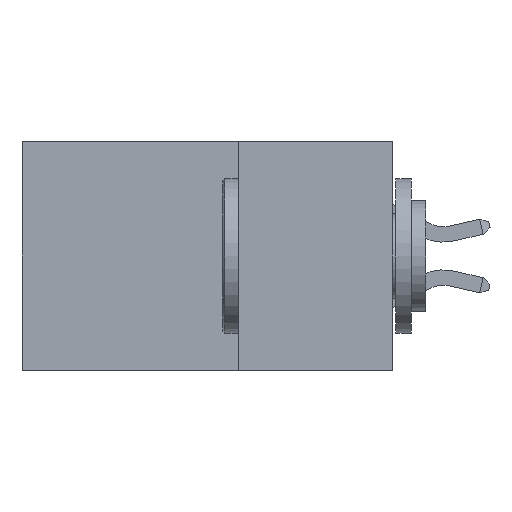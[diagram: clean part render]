
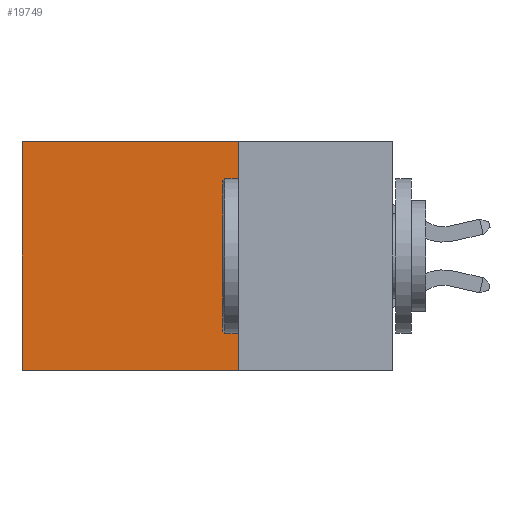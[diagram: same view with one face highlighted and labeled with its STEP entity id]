
A CAD part, left-side view. The second image highlights one B-rep face of the part: STEP entity #19749.
In plain terms, the highlighted planar face has unit normal (-1, 0, 0).
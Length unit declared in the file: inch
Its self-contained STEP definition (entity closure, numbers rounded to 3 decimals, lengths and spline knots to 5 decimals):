
#245 = LINE ( 'NONE', #20423, #14834 ) ;
#552 = CARTESIAN_POINT ( 'NONE',  ( 0.2875, 0.25, 0. ) ) ;
#1930 = DIRECTION ( 'NONE',  ( 0., 0., -1. ) ) ;
#2549 = CARTESIAN_POINT ( 'NONE',  ( 0.2875, 0.6, -0.37 ) ) ;
#3385 = EDGE_CURVE ( 'NONE', #13468, #19753, #19648, .T. ) ;
#4833 = EDGE_CURVE ( 'NONE', #16592, #5037, #22550, .T. ) ;
#4942 = DIRECTION ( 'NONE',  ( 0., 1., 0. ) ) ;
#5016 = EDGE_CURVE ( 'NONE', #13468, #16592, #245, .T. ) ;
#5037 = VERTEX_POINT ( 'NONE', #2549 ) ;
#5762 = DIRECTION ( 'NONE',  ( 1., 0., 0. ) ) ;
#8486 = DIRECTION ( 'NONE',  ( 0., 0., -1. ) ) ;
#8752 = CARTESIAN_POINT ( 'NONE',  ( 0.2875, 0.6, 0. ) ) ;
#9355 = VECTOR ( 'NONE', #14671, 39.37008 ) ;
#9581 = CARTESIAN_POINT ( 'NONE',  ( 0.2875, 0.25, 0. ) ) ;
#11023 = ORIENTED_EDGE ( 'NONE', *, *, #5016, .T. ) ;
#12204 = CARTESIAN_POINT ( 'NONE',  ( 0.2875, 0.25, -0.37 ) ) ;
#12435 = CARTESIAN_POINT ( 'NONE',  ( 0.2875, 0.6, 0. ) ) ;
#13152 = ORIENTED_EDGE ( 'NONE', *, *, #3385, .F. ) ;
#13156 = CARTESIAN_POINT ( 'NONE',  ( 0.2875, 0.25, -0.37 ) ) ;
#13258 = VECTOR ( 'NONE', #8486, 39.37008 ) ;
#13468 = VERTEX_POINT ( 'NONE', #552 ) ;
#14671 = DIRECTION ( 'NONE',  ( 0., 1., 0. ) ) ;
#14834 = VECTOR ( 'NONE', #4942, 39.37008 ) ;
#15577 = VECTOR ( 'NONE', #20568, 39.37008 ) ;
#16141 = CARTESIAN_POINT ( 'NONE',  ( 0.2875, 0.25, 0. ) ) ;
#16592 = VERTEX_POINT ( 'NONE', #8752 ) ;
#16826 = AXIS2_PLACEMENT_3D ( 'NONE', #9581, #5762, #1930 ) ;
#17412 = ORIENTED_EDGE ( 'NONE', *, *, #23725, .F. ) ;
#18948 = LINE ( 'NONE', #12204, #9355 ) ;
#18951 = ORIENTED_EDGE ( 'NONE', *, *, #4833, .T. ) ;
#19648 = LINE ( 'NONE', #16141, #13258 ) ;
#19749 = ADVANCED_FACE ( 'NONE', ( #21705 ), #22422, .F. ) ;
#19753 = VERTEX_POINT ( 'NONE', #13156 ) ;
#20423 = CARTESIAN_POINT ( 'NONE',  ( 0.2875, 0.25, 0. ) ) ;
#20568 = DIRECTION ( 'NONE',  ( 0., 0., -1. ) ) ;
#21705 = FACE_OUTER_BOUND ( 'NONE', #24094, .T. ) ;
#22422 = PLANE ( 'NONE',  #16826 ) ;
#22550 = LINE ( 'NONE', #12435, #15577 ) ;
#23725 = EDGE_CURVE ( 'NONE', #19753, #5037, #18948, .T. ) ;
#24094 = EDGE_LOOP ( 'NONE', ( #18951, #17412, #13152, #11023 ) ) ;
